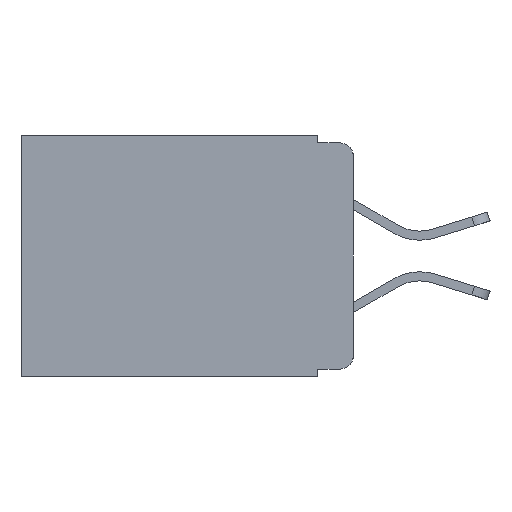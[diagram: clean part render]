
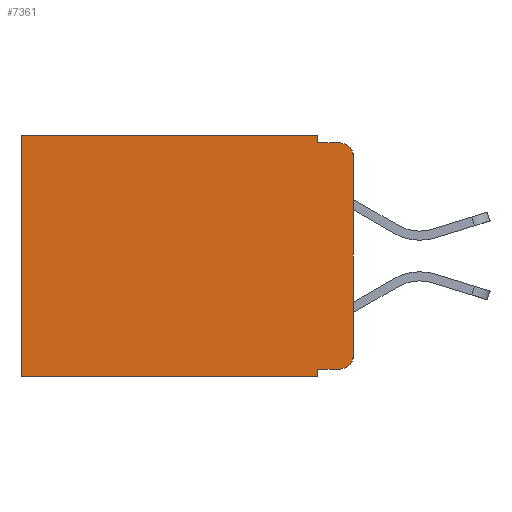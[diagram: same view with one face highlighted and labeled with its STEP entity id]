
A CAD part, left-side view. The second image highlights one B-rep face of the part: STEP entity #7361.
In plain terms, the highlighted planar face has unit normal (-1, 0, 0).
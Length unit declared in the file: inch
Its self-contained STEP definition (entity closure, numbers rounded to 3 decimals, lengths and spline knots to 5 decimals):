
#216 = CARTESIAN_POINT ( 'NONE',  ( 0.298, 0.02, -0.03 ) ) ;
#248 = DIRECTION ( 'NONE',  ( 0., 1., 0. ) ) ;
#276 = ORIENTED_EDGE ( 'NONE', *, *, #3625, .T. ) ;
#521 = EDGE_CURVE ( 'NONE', #8392, #3568, #1773, .T. ) ;
#798 = VECTOR ( 'NONE', #4860, 39.37008 ) ;
#817 = VERTEX_POINT ( 'NONE', #12078 ) ;
#1129 = DIRECTION ( 'NONE',  ( 0., 0., -1. ) ) ;
#1141 = VERTEX_POINT ( 'NONE', #15442 ) ;
#1448 = FACE_OUTER_BOUND ( 'NONE', #12434, .T. ) ;
#1499 = CARTESIAN_POINT ( 'NONE',  ( 0.298, 0.02, -0.01 ) ) ;
#1626 = CARTESIAN_POINT ( 'NONE',  ( 0.298, 0.02, -0.313 ) ) ;
#1773 = LINE ( 'NONE', #12213, #13241 ) ;
#2154 = VECTOR ( 'NONE', #8763, 39.37008 ) ;
#2613 = CARTESIAN_POINT ( 'NONE',  ( 0.298, 0.051, -0.01 ) ) ;
#3066 = DIRECTION ( 'NONE',  ( 0., 0., -1. ) ) ;
#3150 = CARTESIAN_POINT ( 'NONE',  ( 0.298, 0.051, 0. ) ) ;
#3472 = DIRECTION ( 'NONE',  ( 0., -1., 0. ) ) ;
#3526 = CARTESIAN_POINT ( 'NONE',  ( 0.298, 0.473, -0.343 ) ) ;
#3568 = VERTEX_POINT ( 'NONE', #13758 ) ;
#3625 = EDGE_CURVE ( 'NONE', #8764, #3646, #9270, .T. ) ;
#3646 = VERTEX_POINT ( 'NONE', #1499 ) ;
#3891 = VECTOR ( 'NONE', #9005, 39.37008 ) ;
#4246 = ORIENTED_EDGE ( 'NONE', *, *, #9959, .F. ) ;
#4261 = ORIENTED_EDGE ( 'NONE', *, *, #14744, .F. ) ;
#4860 = DIRECTION ( 'NONE',  ( 0., 1., 0. ) ) ;
#5019 = CARTESIAN_POINT ( 'NONE',  ( 0.298, 0.051, -0.01 ) ) ;
#5271 = DIRECTION ( 'NONE',  ( 0., 0., -1. ) ) ;
#5454 = CARTESIAN_POINT ( 'NONE',  ( 0.298, 0., 0. ) ) ;
#5604 = VECTOR ( 'NONE', #5271, 39.37008 ) ;
#6082 = LINE ( 'NONE', #16611, #13326 ) ;
#6225 = DIRECTION ( 'NONE',  ( 0., 0., -1. ) ) ;
#6251 = EDGE_CURVE ( 'NONE', #9934, #3646, #7662, .T. ) ;
#6829 = LINE ( 'NONE', #3150, #2154 ) ;
#6939 = DIRECTION ( 'NONE',  ( 0., 0., -1. ) ) ;
#7154 = AXIS2_PLACEMENT_3D ( 'NONE', #1626, #11364, #3066 ) ;
#7174 = EDGE_CURVE ( 'NONE', #9051, #7205, #15382, .T. ) ;
#7205 = VERTEX_POINT ( 'NONE', #3526 ) ;
#7361 = ADVANCED_FACE ( 'NONE', ( #1448 ), #7823, .F. ) ;
#7662 = LINE ( 'NONE', #5019, #3891 ) ;
#7823 = PLANE ( 'NONE',  #9435 ) ;
#8392 = VERTEX_POINT ( 'NONE', #11786 ) ;
#8662 = ORIENTED_EDGE ( 'NONE', *, *, #6251, .F. ) ;
#8763 = DIRECTION ( 'NONE',  ( 0., 0., -1. ) ) ;
#8764 = VERTEX_POINT ( 'NONE', #11220 ) ;
#9005 = DIRECTION ( 'NONE',  ( 0., -1., 0. ) ) ;
#9030 = EDGE_CURVE ( 'NONE', #8392, #9051, #14517, .T. ) ;
#9051 = VERTEX_POINT ( 'NONE', #15682 ) ;
#9113 = CIRCLE ( 'NONE', #7154, 0.02 ) ;
#9210 = DIRECTION ( 'NONE',  ( 0., 0., -1. ) ) ;
#9270 = CIRCLE ( 'NONE', #13415, 0.02 ) ;
#9435 = AXIS2_PLACEMENT_3D ( 'NONE', #15462, #17073, #9210 ) ;
#9934 = VERTEX_POINT ( 'NONE', #2613 ) ;
#9959 = EDGE_CURVE ( 'NONE', #8764, #817, #15365, .T. ) ;
#10132 = EDGE_CURVE ( 'NONE', #1141, #16696, #6082, .T. ) ;
#10143 = ORIENTED_EDGE ( 'NONE', *, *, #521, .T. ) ;
#10385 = CARTESIAN_POINT ( 'NONE',  ( 0.298, 0.051, 0. ) ) ;
#10556 = VECTOR ( 'NONE', #6225, 39.37008 ) ;
#10558 = ORIENTED_EDGE ( 'NONE', *, *, #9030, .F. ) ;
#11152 = DIRECTION ( 'NONE',  ( -1., 0., 0. ) ) ;
#11220 = CARTESIAN_POINT ( 'NONE',  ( 0.298, 0., -0.03 ) ) ;
#11364 = DIRECTION ( 'NONE',  ( -1., 0., 0. ) ) ;
#11643 = EDGE_CURVE ( 'NONE', #16696, #7205, #12463, .T. ) ;
#11786 = CARTESIAN_POINT ( 'NONE',  ( 0.298, 0.051, -0.333 ) ) ;
#11867 = VECTOR ( 'NONE', #6939, 39.37008 ) ;
#12021 = ORIENTED_EDGE ( 'NONE', *, *, #7174, .F. ) ;
#12078 = CARTESIAN_POINT ( 'NONE',  ( 0.298, 0., -0.313 ) ) ;
#12213 = CARTESIAN_POINT ( 'NONE',  ( 0.298, 0.051, -0.333 ) ) ;
#12434 = EDGE_LOOP ( 'NONE', ( #4246, #276, #8662, #4261, #15506, #15321, #12021, #10558, #10143, #17506 ) ) ;
#12463 = LINE ( 'NONE', #14778, #5604 ) ;
#13241 = VECTOR ( 'NONE', #3472, 39.37008 ) ;
#13272 = CARTESIAN_POINT ( 'NONE',  ( 0.298, 0.473, 0. ) ) ;
#13326 = VECTOR ( 'NONE', #248, 39.37008 ) ;
#13415 = AXIS2_PLACEMENT_3D ( 'NONE', #216, #11152, #1129 ) ;
#13758 = CARTESIAN_POINT ( 'NONE',  ( 0.298, 0.02, -0.333 ) ) ;
#14395 = CARTESIAN_POINT ( 'NONE',  ( 0.298, 0., -0.343 ) ) ;
#14517 = LINE ( 'NONE', #10385, #10556 ) ;
#14744 = EDGE_CURVE ( 'NONE', #1141, #9934, #6829, .T. ) ;
#14778 = CARTESIAN_POINT ( 'NONE',  ( 0.298, 0.473, 0. ) ) ;
#15321 = ORIENTED_EDGE ( 'NONE', *, *, #11643, .T. ) ;
#15365 = LINE ( 'NONE', #5454, #11867 ) ;
#15382 = LINE ( 'NONE', #14395, #798 ) ;
#15442 = CARTESIAN_POINT ( 'NONE',  ( 0.298, 0.051, 0. ) ) ;
#15462 = CARTESIAN_POINT ( 'NONE',  ( 0.298, 0., 0. ) ) ;
#15506 = ORIENTED_EDGE ( 'NONE', *, *, #10132, .T. ) ;
#15682 = CARTESIAN_POINT ( 'NONE',  ( 0.298, 0.051, -0.343 ) ) ;
#15788 = EDGE_CURVE ( 'NONE', #3568, #817, #9113, .T. ) ;
#16611 = CARTESIAN_POINT ( 'NONE',  ( 0.298, 0., 0. ) ) ;
#16696 = VERTEX_POINT ( 'NONE', #13272 ) ;
#17073 = DIRECTION ( 'NONE',  ( 1., 0., 0. ) ) ;
#17506 = ORIENTED_EDGE ( 'NONE', *, *, #15788, .T. ) ;
